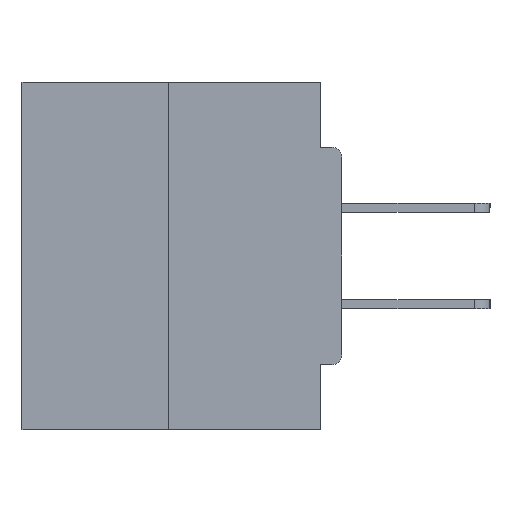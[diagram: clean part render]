
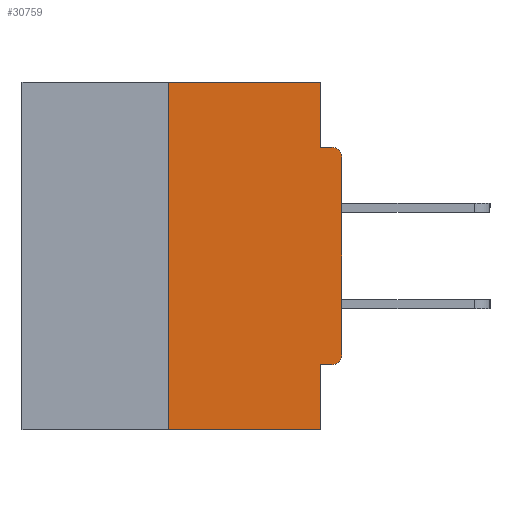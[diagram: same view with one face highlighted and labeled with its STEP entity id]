
A CAD part, left-side view. The second image highlights one B-rep face of the part: STEP entity #30759.
In plain terms, the highlighted planar face has unit normal (-1, 0, 0).
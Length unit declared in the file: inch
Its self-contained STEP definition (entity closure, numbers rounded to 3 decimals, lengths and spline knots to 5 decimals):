
#262 = PLANE ( 'NONE',  #34924 ) ;
#358 = DIRECTION ( 'NONE',  ( 0., 0., -1. ) ) ;
#646 = EDGE_CURVE ( 'NONE', #14703, #31935, #1647, .T. ) ;
#789 = CARTESIAN_POINT ( 'NONE',  ( 0., 0.031, 0. ) ) ;
#807 = DIRECTION ( 'NONE',  ( 0., 1., 0. ) ) ;
#1462 = VECTOR ( 'NONE', #28649, 39.37008 ) ;
#1647 = LINE ( 'NONE', #36015, #5176 ) ;
#2046 = VERTEX_POINT ( 'NONE', #23749 ) ;
#2616 = LINE ( 'NONE', #26065, #17035 ) ;
#3760 = VERTEX_POINT ( 'NONE', #35118 ) ;
#3820 = ORIENTED_EDGE ( 'NONE', *, *, #33928, .F. ) ;
#4780 = CARTESIAN_POINT ( 'NONE',  ( 0., 0., -0.3915 ) ) ;
#4789 = VERTEX_POINT ( 'NONE', #34011 ) ;
#5176 = VECTOR ( 'NONE', #21710, 39.37008 ) ;
#5901 = ORIENTED_EDGE ( 'NONE', *, *, #19874, .F. ) ;
#6091 = CARTESIAN_POINT ( 'NONE',  ( 0., 0., -0.0935 ) ) ;
#6166 = LINE ( 'NONE', #8966, #18831 ) ;
#6456 = EDGE_LOOP ( 'NONE', ( #3820, #22237, #30655, #5901, #33952, #10186, #20639, #9250, #18281, #10532 ) ) ;
#7596 = EDGE_CURVE ( 'NONE', #3760, #4789, #15064, .T. ) ;
#8438 = VERTEX_POINT ( 'NONE', #18426 ) ;
#8966 = CARTESIAN_POINT ( 'NONE',  ( 0., 0.46, -0.5 ) ) ;
#9250 = ORIENTED_EDGE ( 'NONE', *, *, #13785, .T. ) ;
#10186 = ORIENTED_EDGE ( 'NONE', *, *, #20452, .T. ) ;
#10492 = CIRCLE ( 'NONE', #26055, 0.015 ) ;
#10532 = ORIENTED_EDGE ( 'NONE', *, *, #26081, .F. ) ;
#11513 = CARTESIAN_POINT ( 'NONE',  ( 0., 0., -0.1085 ) ) ;
#12626 = EDGE_CURVE ( 'NONE', #8438, #15196, #6166, .T. ) ;
#13482 = CARTESIAN_POINT ( 'NONE',  ( 0., 0.015, -0.3915 ) ) ;
#13785 = EDGE_CURVE ( 'NONE', #31935, #35903, #10492, .T. ) ;
#14582 = LINE ( 'NONE', #31505, #23005 ) ;
#14703 = VERTEX_POINT ( 'NONE', #4780 ) ;
#14920 = LINE ( 'NONE', #6091, #1462 ) ;
#15064 = LINE ( 'NONE', #26525, #31849 ) ;
#15196 = VERTEX_POINT ( 'NONE', #28729 ) ;
#15456 = VECTOR ( 'NONE', #20368, 39.37008 ) ;
#16302 = VERTEX_POINT ( 'NONE', #789 ) ;
#16672 = DIRECTION ( 'NONE',  ( -1., 0., 0. ) ) ;
#17035 = VECTOR ( 'NONE', #358, 39.37008 ) ;
#17921 = LINE ( 'NONE', #21102, #15456 ) ;
#18180 = CARTESIAN_POINT ( 'NONE',  ( 0., 0.031, -0.0935 ) ) ;
#18281 = ORIENTED_EDGE ( 'NONE', *, *, #35673, .F. ) ;
#18426 = CARTESIAN_POINT ( 'NONE',  ( 0., 0.25, -0.5 ) ) ;
#18831 = VECTOR ( 'NONE', #19197, 39.37008 ) ;
#19197 = DIRECTION ( 'NONE',  ( 0., -1., 0. ) ) ;
#19874 = EDGE_CURVE ( 'NONE', #4789, #15196, #2616, .T. ) ;
#20368 = DIRECTION ( 'NONE',  ( 0., 0., -1. ) ) ;
#20452 = EDGE_CURVE ( 'NONE', #3760, #14703, #29702, .T. ) ;
#20520 = DIRECTION ( 'NONE',  ( 1., 0., 0. ) ) ;
#20639 = ORIENTED_EDGE ( 'NONE', *, *, #646, .T. ) ;
#21102 = CARTESIAN_POINT ( 'NONE',  ( 0., 0.031, 0. ) ) ;
#21710 = DIRECTION ( 'NONE',  ( 0., 0., 1. ) ) ;
#22237 = ORIENTED_EDGE ( 'NONE', *, *, #23026, .F. ) ;
#22964 = CARTESIAN_POINT ( 'NONE',  ( 0., 0.46, 0. ) ) ;
#23005 = VECTOR ( 'NONE', #26037, 39.37008 ) ;
#23026 = EDGE_CURVE ( 'NONE', #8438, #2046, #25697, .T. ) ;
#23051 = CARTESIAN_POINT ( 'NONE',  ( 0., 0.25, 0. ) ) ;
#23749 = CARTESIAN_POINT ( 'NONE',  ( 0., 0.25, 0. ) ) ;
#24929 = AXIS2_PLACEMENT_3D ( 'NONE', #13482, #16672, #25134 ) ;
#25134 = DIRECTION ( 'NONE',  ( 0., 0., -1. ) ) ;
#25697 = LINE ( 'NONE', #23051, #35696 ) ;
#26037 = DIRECTION ( 'NONE',  ( 0., -1., 0. ) ) ;
#26055 = AXIS2_PLACEMENT_3D ( 'NONE', #27657, #30306, #29921 ) ;
#26065 = CARTESIAN_POINT ( 'NONE',  ( 0., 0.031, -0.5 ) ) ;
#26081 = EDGE_CURVE ( 'NONE', #16302, #36737, #17921, .T. ) ;
#26525 = CARTESIAN_POINT ( 'NONE',  ( 0., 0., -0.4065 ) ) ;
#27657 = CARTESIAN_POINT ( 'NONE',  ( 0., 0.015, -0.1085 ) ) ;
#28633 = FACE_OUTER_BOUND ( 'NONE', #6456, .T. ) ;
#28649 = DIRECTION ( 'NONE',  ( 0., -1., 0. ) ) ;
#28729 = CARTESIAN_POINT ( 'NONE',  ( 0., 0.031, -0.5 ) ) ;
#29192 = DIRECTION ( 'NONE',  ( 0., 0., -1. ) ) ;
#29702 = CIRCLE ( 'NONE', #24929, 0.015 ) ;
#29758 = CARTESIAN_POINT ( 'NONE',  ( 0., 0.015, -0.0935 ) ) ;
#29921 = DIRECTION ( 'NONE',  ( 0., 0., -1. ) ) ;
#30306 = DIRECTION ( 'NONE',  ( -1., 0., 0. ) ) ;
#30655 = ORIENTED_EDGE ( 'NONE', *, *, #12626, .T. ) ;
#30759 = ADVANCED_FACE ( 'NONE', ( #28633 ), #262, .F. ) ;
#31505 = CARTESIAN_POINT ( 'NONE',  ( 0., 0.46, 0. ) ) ;
#31710 = DIRECTION ( 'NONE',  ( 0., 0., 1. ) ) ;
#31849 = VECTOR ( 'NONE', #807, 39.37008 ) ;
#31935 = VERTEX_POINT ( 'NONE', #11513 ) ;
#33928 = EDGE_CURVE ( 'NONE', #2046, #16302, #14582, .T. ) ;
#33952 = ORIENTED_EDGE ( 'NONE', *, *, #7596, .F. ) ;
#34011 = CARTESIAN_POINT ( 'NONE',  ( 0., 0.031, -0.4065 ) ) ;
#34924 = AXIS2_PLACEMENT_3D ( 'NONE', #22964, #20520, #29192 ) ;
#35118 = CARTESIAN_POINT ( 'NONE',  ( 0., 0.015, -0.4065 ) ) ;
#35673 = EDGE_CURVE ( 'NONE', #36737, #35903, #14920, .T. ) ;
#35696 = VECTOR ( 'NONE', #31710, 39.37008 ) ;
#35903 = VERTEX_POINT ( 'NONE', #29758 ) ;
#36015 = CARTESIAN_POINT ( 'NONE',  ( 0., 0., 0. ) ) ;
#36737 = VERTEX_POINT ( 'NONE', #18180 ) ;
